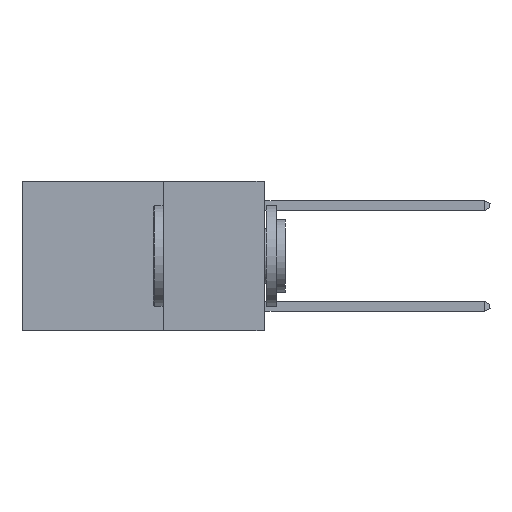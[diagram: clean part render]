
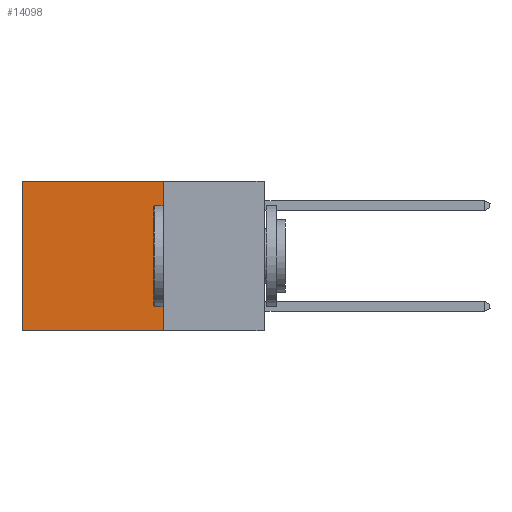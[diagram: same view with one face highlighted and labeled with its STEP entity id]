
A CAD part, left-side view. The second image highlights one B-rep face of the part: STEP entity #14098.
In plain terms, the highlighted planar face has unit normal (-1, 0, 0).
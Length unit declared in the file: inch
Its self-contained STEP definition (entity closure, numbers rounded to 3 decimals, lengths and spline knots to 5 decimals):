
#119 = CARTESIAN_POINT ( 'NONE',  ( 0.2625, 0.25, -0.37 ) ) ;
#290 = CARTESIAN_POINT ( 'NONE',  ( 0.2625, 0.25, -0.37 ) ) ;
#397 = DIRECTION ( 'NONE',  ( 0., 0., -1. ) ) ;
#609 = CARTESIAN_POINT ( 'NONE',  ( 0.2625, 0.25, 0. ) ) ;
#715 = VECTOR ( 'NONE', #6875, 39.37008 ) ;
#1131 = DIRECTION ( 'NONE',  ( 0., 1., 0. ) ) ;
#1240 = CARTESIAN_POINT ( 'NONE',  ( 0.2625, 0.6, 0. ) ) ;
#1537 = PLANE ( 'NONE',  #2447 ) ;
#1637 = VERTEX_POINT ( 'NONE', #13401 ) ;
#1680 = FACE_OUTER_BOUND ( 'NONE', #12266, .T. ) ;
#2062 = VERTEX_POINT ( 'NONE', #3050 ) ;
#2447 = AXIS2_PLACEMENT_3D ( 'NONE', #609, #13160, #397 ) ;
#2622 = ORIENTED_EDGE ( 'NONE', *, *, #4569, .F. ) ;
#3050 = CARTESIAN_POINT ( 'NONE',  ( 0.2625, 0.6, -0.37 ) ) ;
#3071 = LINE ( 'NONE', #8940, #4368 ) ;
#3364 = VECTOR ( 'NONE', #14121, 39.37008 ) ;
#3674 = VERTEX_POINT ( 'NONE', #13225 ) ;
#4368 = VECTOR ( 'NONE', #13625, 39.37008 ) ;
#4569 = EDGE_CURVE ( 'NONE', #6948, #2062, #13323, .T. ) ;
#5552 = CARTESIAN_POINT ( 'NONE',  ( 0.2625, 0.25, 0. ) ) ;
#6875 = DIRECTION ( 'NONE',  ( 0., 0., -1. ) ) ;
#6948 = VERTEX_POINT ( 'NONE', #290 ) ;
#7284 = ORIENTED_EDGE ( 'NONE', *, *, #8018, .T. ) ;
#8018 = EDGE_CURVE ( 'NONE', #3674, #1637, #12588, .T. ) ;
#8940 = CARTESIAN_POINT ( 'NONE',  ( 0.2625, 0.25, 0. ) ) ;
#9394 = LINE ( 'NONE', #1240, #715 ) ;
#9636 = ORIENTED_EDGE ( 'NONE', *, *, #13059, .T. ) ;
#12266 = EDGE_LOOP ( 'NONE', ( #9636, #2622, #14006, #7284 ) ) ;
#12588 = LINE ( 'NONE', #5552, #13837 ) ;
#12952 = EDGE_CURVE ( 'NONE', #3674, #6948, #3071, .T. ) ;
#13059 = EDGE_CURVE ( 'NONE', #1637, #2062, #9394, .T. ) ;
#13160 = DIRECTION ( 'NONE',  ( 1., 0., 0. ) ) ;
#13225 = CARTESIAN_POINT ( 'NONE',  ( 0.2625, 0.25, 0. ) ) ;
#13323 = LINE ( 'NONE', #119, #3364 ) ;
#13401 = CARTESIAN_POINT ( 'NONE',  ( 0.2625, 0.6, 0. ) ) ;
#13625 = DIRECTION ( 'NONE',  ( 0., 0., -1. ) ) ;
#13837 = VECTOR ( 'NONE', #1131, 39.37008 ) ;
#14006 = ORIENTED_EDGE ( 'NONE', *, *, #12952, .F. ) ;
#14098 = ADVANCED_FACE ( 'NONE', ( #1680 ), #1537, .F. ) ;
#14121 = DIRECTION ( 'NONE',  ( 0., 1., 0. ) ) ;
